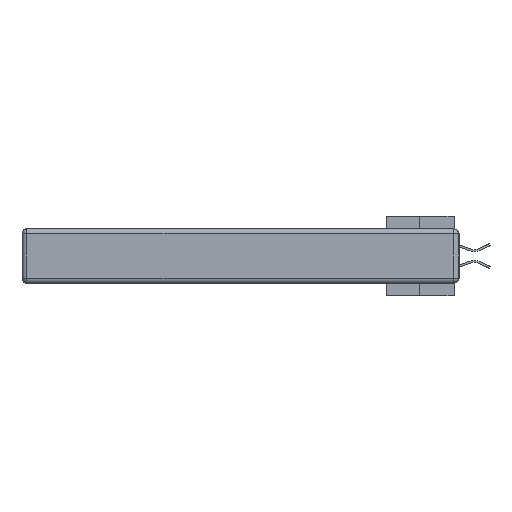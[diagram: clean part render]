
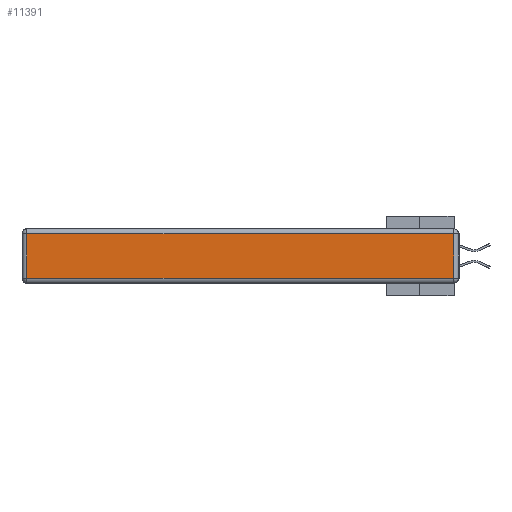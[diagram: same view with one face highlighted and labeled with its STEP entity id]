
A CAD part, left-side view. The second image highlights one B-rep face of the part: STEP entity #11391.
In plain terms, the highlighted planar face has unit normal (-1, 0, 0).
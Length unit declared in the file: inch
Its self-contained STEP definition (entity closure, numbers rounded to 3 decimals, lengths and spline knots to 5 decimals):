
#1285 = DIRECTION ( 'NONE',  ( 0., -1., 0. ) ) ;
#1306 = ORIENTED_EDGE ( 'NONE', *, *, #28716, .T. ) ;
#2173 = ORIENTED_EDGE ( 'NONE', *, *, #11364, .T. ) ;
#2442 = VERTEX_POINT ( 'NONE', #6772 ) ;
#2662 = VERTEX_POINT ( 'NONE', #34666 ) ;
#4403 = EDGE_CURVE ( 'NONE', #2442, #30493, #29412, .T. ) ;
#6772 = CARTESIAN_POINT ( 'NONE',  ( 0., 2.72, -0.313 ) ) ;
#7621 = LINE ( 'NONE', #20355, #30919 ) ;
#7630 = VECTOR ( 'NONE', #19334, 39.37008 ) ;
#7634 = LINE ( 'NONE', #9588, #8899 ) ;
#7773 = EDGE_LOOP ( 'NONE', ( #30669, #1306, #2173, #10730 ) ) ;
#8899 = VECTOR ( 'NONE', #12323, 39.37008 ) ;
#9588 = CARTESIAN_POINT ( 'NONE',  ( 0., 2.72, -0.343 ) ) ;
#10730 = ORIENTED_EDGE ( 'NONE', *, *, #32044, .T. ) ;
#10782 = VECTOR ( 'NONE', #1285, 39.37008 ) ;
#11364 = EDGE_CURVE ( 'NONE', #2662, #34824, #22068, .T. ) ;
#11391 = ADVANCED_FACE ( 'NONE', ( #12740 ), #16251, .T. ) ;
#12323 = DIRECTION ( 'NONE',  ( 0., 0., -1. ) ) ;
#12740 = FACE_OUTER_BOUND ( 'NONE', #7773, .T. ) ;
#13515 = CARTESIAN_POINT ( 'NONE',  ( 0., 2.75, -0.03 ) ) ;
#16251 = PLANE ( 'NONE',  #17880 ) ;
#16653 = CARTESIAN_POINT ( 'NONE',  ( 0., 0., -0.313 ) ) ;
#17880 = AXIS2_PLACEMENT_3D ( 'NONE', #21598, #18999, #24547 ) ;
#18999 = DIRECTION ( 'NONE',  ( -1., 0., 0. ) ) ;
#19334 = DIRECTION ( 'NONE',  ( 0., 1., 0. ) ) ;
#20355 = CARTESIAN_POINT ( 'NONE',  ( 0., 0.03, -0.343 ) ) ;
#21598 = CARTESIAN_POINT ( 'NONE',  ( 0., 0., -0.343 ) ) ;
#22068 = LINE ( 'NONE', #13515, #7630 ) ;
#22298 = CARTESIAN_POINT ( 'NONE',  ( 0., 2.72, -0.03 ) ) ;
#23182 = CARTESIAN_POINT ( 'NONE',  ( 0., 0.03, -0.313 ) ) ;
#24547 = DIRECTION ( 'NONE',  ( 0., 0., 1. ) ) ;
#25760 = DIRECTION ( 'NONE',  ( 0., 0., 1. ) ) ;
#28716 = EDGE_CURVE ( 'NONE', #30493, #2662, #7621, .T. ) ;
#29412 = LINE ( 'NONE', #16653, #10782 ) ;
#30493 = VERTEX_POINT ( 'NONE', #23182 ) ;
#30669 = ORIENTED_EDGE ( 'NONE', *, *, #4403, .T. ) ;
#30919 = VECTOR ( 'NONE', #25760, 39.37008 ) ;
#32044 = EDGE_CURVE ( 'NONE', #34824, #2442, #7634, .T. ) ;
#34666 = CARTESIAN_POINT ( 'NONE',  ( 0., 0.03, -0.03 ) ) ;
#34824 = VERTEX_POINT ( 'NONE', #22298 ) ;
